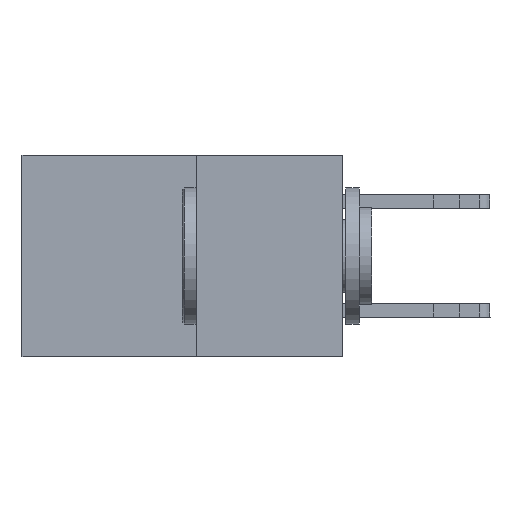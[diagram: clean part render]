
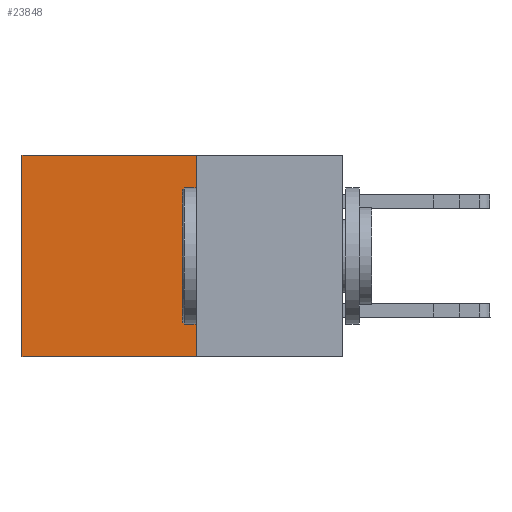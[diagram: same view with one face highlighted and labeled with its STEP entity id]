
A CAD part, left-side view. The second image highlights one B-rep face of the part: STEP entity #23848.
In plain terms, the highlighted planar face has unit normal (-1, 0, 0).
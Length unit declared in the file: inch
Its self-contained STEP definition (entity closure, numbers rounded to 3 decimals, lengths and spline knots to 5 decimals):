
#521 = VERTEX_POINT ( 'NONE', #18524 ) ;
#696 = CARTESIAN_POINT ( 'NONE',  ( 0.277, 0.27, -0.37 ) ) ;
#1809 = DIRECTION ( 'NONE',  ( 0., 1., 0. ) ) ;
#2148 = EDGE_CURVE ( 'NONE', #521, #18671, #14967, .T. ) ;
#2251 = VECTOR ( 'NONE', #7419, 39.37008 ) ;
#2511 = PLANE ( 'NONE',  #23903 ) ;
#2668 = ORIENTED_EDGE ( 'NONE', *, *, #6640, .F. ) ;
#4620 = DIRECTION ( 'NONE',  ( 1., 0., 0. ) ) ;
#4791 = FACE_OUTER_BOUND ( 'NONE', #8705, .T. ) ;
#4878 = EDGE_CURVE ( 'NONE', #521, #13531, #10493, .T. ) ;
#6614 = CARTESIAN_POINT ( 'NONE',  ( 0.277, 0.59, -0.37 ) ) ;
#6640 = EDGE_CURVE ( 'NONE', #18671, #20555, #22294, .T. ) ;
#7007 = LINE ( 'NONE', #19387, #2251 ) ;
#7419 = DIRECTION ( 'NONE',  ( 0., 0., -1. ) ) ;
#8185 = CARTESIAN_POINT ( 'NONE',  ( 0.277, 0.59, 0. ) ) ;
#8396 = ORIENTED_EDGE ( 'NONE', *, *, #10349, .T. ) ;
#8705 = EDGE_LOOP ( 'NONE', ( #8396, #2668, #14105, #16240 ) ) ;
#9080 = CARTESIAN_POINT ( 'NONE',  ( 0.277, 0.27, -0.37 ) ) ;
#9661 = VECTOR ( 'NONE', #11448, 39.37008 ) ;
#10349 = EDGE_CURVE ( 'NONE', #13531, #20555, #7007, .T. ) ;
#10493 = LINE ( 'NONE', #11816, #20505 ) ;
#11448 = DIRECTION ( 'NONE',  ( 0., 0., -1. ) ) ;
#11731 = DIRECTION ( 'NONE',  ( 0., 1., 0. ) ) ;
#11816 = CARTESIAN_POINT ( 'NONE',  ( 0.277, 0.27, 0. ) ) ;
#12582 = CARTESIAN_POINT ( 'NONE',  ( 0.277, 0.27, -0.37 ) ) ;
#13531 = VERTEX_POINT ( 'NONE', #8185 ) ;
#13799 = CARTESIAN_POINT ( 'NONE',  ( 0.277, 0.27, -0.37 ) ) ;
#14105 = ORIENTED_EDGE ( 'NONE', *, *, #2148, .F. ) ;
#14967 = LINE ( 'NONE', #13799, #9661 ) ;
#16240 = ORIENTED_EDGE ( 'NONE', *, *, #4878, .T. ) ;
#17592 = VECTOR ( 'NONE', #1809, 39.37008 ) ;
#18524 = CARTESIAN_POINT ( 'NONE',  ( 0.277, 0.27, 0. ) ) ;
#18630 = DIRECTION ( 'NONE',  ( 0., 0., -1. ) ) ;
#18671 = VERTEX_POINT ( 'NONE', #9080 ) ;
#19387 = CARTESIAN_POINT ( 'NONE',  ( 0.277, 0.59, -0.37 ) ) ;
#20505 = VECTOR ( 'NONE', #11731, 39.37008 ) ;
#20555 = VERTEX_POINT ( 'NONE', #6614 ) ;
#22294 = LINE ( 'NONE', #696, #17592 ) ;
#23848 = ADVANCED_FACE ( 'NONE', ( #4791 ), #2511, .F. ) ;
#23903 = AXIS2_PLACEMENT_3D ( 'NONE', #12582, #4620, #18630 ) ;
